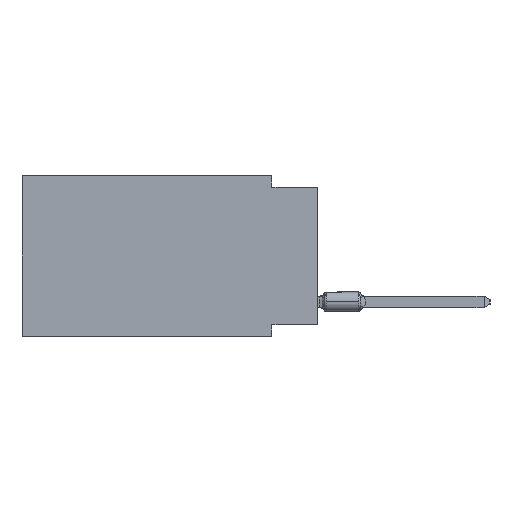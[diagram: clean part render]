
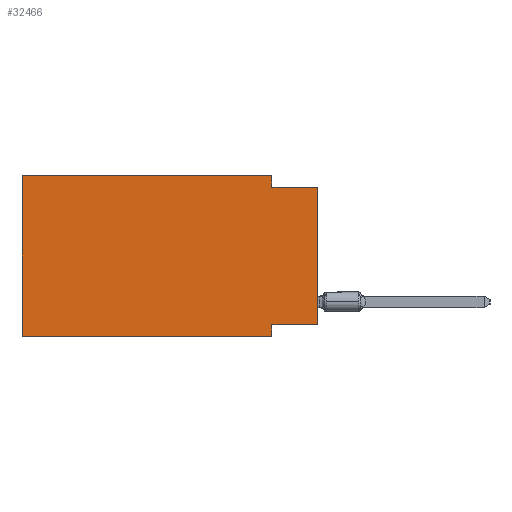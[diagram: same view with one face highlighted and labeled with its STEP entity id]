
A CAD part, left-side view. The second image highlights one B-rep face of the part: STEP entity #32466.
In plain terms, the highlighted planar face has unit normal (-1, 0, 0).
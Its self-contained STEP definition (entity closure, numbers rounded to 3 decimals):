
#559 = AXIS2_PLACEMENT_3D ( 'NONE', #15030, #29965, #12486 ) ;
#1690 = EDGE_CURVE ( 'NONE', #4900, #24685, #18037, .T. ) ;
#1785 = DIRECTION ( 'NONE',  ( 0., 0., -1. ) ) ;
#2520 = VECTOR ( 'NONE', #30578, 1000. ) ;
#2607 = LINE ( 'NONE', #26050, #9326 ) ;
#3998 = VERTEX_POINT ( 'NONE', #26127 ) ;
#4900 = VERTEX_POINT ( 'NONE', #22953 ) ;
#5017 = CARTESIAN_POINT ( 'NONE',  ( 0., 2.54, 0. ) ) ;
#5336 = ORIENTED_EDGE ( 'NONE', *, *, #18949, .F. ) ;
#5697 = ORIENTED_EDGE ( 'NONE', *, *, #27160, .T. ) ;
#6663 = DIRECTION ( 'NONE',  ( 0., -1., 0. ) ) ;
#6720 = CARTESIAN_POINT ( 'NONE',  ( 0., 2.54, -8.89 ) ) ;
#8125 = DIRECTION ( 'NONE',  ( 0., 0., 1. ) ) ;
#8494 = CARTESIAN_POINT ( 'NONE',  ( 0., 16.383, -8.89 ) ) ;
#9092 = CARTESIAN_POINT ( 'NONE',  ( 0., 2.54, -0.635 ) ) ;
#9241 = VECTOR ( 'NONE', #1785, 1000. ) ;
#9326 = VECTOR ( 'NONE', #22831, 1000. ) ;
#11205 = CARTESIAN_POINT ( 'NONE',  ( 0., 0., 0. ) ) ;
#11702 = VECTOR ( 'NONE', #21487, 1000. ) ;
#11931 = CARTESIAN_POINT ( 'NONE',  ( 0., 16.383, 0. ) ) ;
#12041 = ORIENTED_EDGE ( 'NONE', *, *, #31662, .F. ) ;
#12143 = PLANE ( 'NONE',  #559 ) ;
#12486 = DIRECTION ( 'NONE',  ( 0., 0., -1. ) ) ;
#14086 = CARTESIAN_POINT ( 'NONE',  ( 0., 0., -8.255 ) ) ;
#15030 = CARTESIAN_POINT ( 'NONE',  ( 0., 16.383, 0. ) ) ;
#15844 = VECTOR ( 'NONE', #6663, 1000. ) ;
#16137 = LINE ( 'NONE', #11205, #31351 ) ;
#16819 = CARTESIAN_POINT ( 'NONE',  ( 0., 2.54, -8.89 ) ) ;
#18037 = LINE ( 'NONE', #6720, #9241 ) ;
#18649 = CARTESIAN_POINT ( 'NONE',  ( 0., 16.383, 0. ) ) ;
#18949 = EDGE_CURVE ( 'NONE', #28218, #4900, #26963, .T. ) ;
#19326 = DIRECTION ( 'NONE',  ( 0., 1., 0. ) ) ;
#19624 = FACE_OUTER_BOUND ( 'NONE', #31236, .T. ) ;
#20350 = CARTESIAN_POINT ( 'NONE',  ( 0., 0., -8.255 ) ) ;
#21392 = DIRECTION ( 'NONE',  ( 0., 0., 1. ) ) ;
#21487 = DIRECTION ( 'NONE',  ( 0., -1., 0. ) ) ;
#21732 = VECTOR ( 'NONE', #19326, 1000. ) ;
#21872 = LINE ( 'NONE', #18649, #27008 ) ;
#22106 = LINE ( 'NONE', #11931, #2520 ) ;
#22497 = VERTEX_POINT ( 'NONE', #5017 ) ;
#22831 = DIRECTION ( 'NONE',  ( 0., 0., -1. ) ) ;
#22953 = CARTESIAN_POINT ( 'NONE',  ( 0., 2.54, -8.255 ) ) ;
#24598 = EDGE_CURVE ( 'NONE', #28218, #3998, #16137, .T. ) ;
#24685 = VERTEX_POINT ( 'NONE', #16819 ) ;
#24711 = CARTESIAN_POINT ( 'NONE',  ( 0., 16.383, -8.89 ) ) ;
#26050 = CARTESIAN_POINT ( 'NONE',  ( 0., 2.54, 0. ) ) ;
#26127 = CARTESIAN_POINT ( 'NONE',  ( 0., 0., -0.635 ) ) ;
#26963 = LINE ( 'NONE', #14086, #21732 ) ;
#27008 = VECTOR ( 'NONE', #8125, 1000. ) ;
#27160 = EDGE_CURVE ( 'NONE', #28047, #24685, #29291, .T. ) ;
#27540 = CARTESIAN_POINT ( 'NONE',  ( 0., 0., -0.635 ) ) ;
#27758 = EDGE_CURVE ( 'NONE', #29347, #22497, #22106, .T. ) ;
#28047 = VERTEX_POINT ( 'NONE', #8494 ) ;
#28129 = ORIENTED_EDGE ( 'NONE', *, *, #24598, .T. ) ;
#28218 = VERTEX_POINT ( 'NONE', #20350 ) ;
#28386 = EDGE_CURVE ( 'NONE', #28047, #29347, #21872, .T. ) ;
#29178 = ORIENTED_EDGE ( 'NONE', *, *, #31325, .F. ) ;
#29252 = ORIENTED_EDGE ( 'NONE', *, *, #28386, .F. ) ;
#29291 = LINE ( 'NONE', #24711, #11702 ) ;
#29347 = VERTEX_POINT ( 'NONE', #30048 ) ;
#29919 = LINE ( 'NONE', #27540, #15844 ) ;
#29965 = DIRECTION ( 'NONE',  ( 1., 0., 0. ) ) ;
#30048 = CARTESIAN_POINT ( 'NONE',  ( 0., 16.383, 0. ) ) ;
#30183 = VERTEX_POINT ( 'NONE', #9092 ) ;
#30578 = DIRECTION ( 'NONE',  ( 0., -1., 0. ) ) ;
#31236 = EDGE_LOOP ( 'NONE', ( #28129, #12041, #29178, #32493, #29252, #5697, #32876, #5336 ) ) ;
#31325 = EDGE_CURVE ( 'NONE', #22497, #30183, #2607, .T. ) ;
#31351 = VECTOR ( 'NONE', #21392, 1000. ) ;
#31662 = EDGE_CURVE ( 'NONE', #30183, #3998, #29919, .T. ) ;
#32466 = ADVANCED_FACE ( 'NONE', ( #19624 ), #12143, .F. ) ;
#32493 = ORIENTED_EDGE ( 'NONE', *, *, #27758, .F. ) ;
#32876 = ORIENTED_EDGE ( 'NONE', *, *, #1690, .F. ) ;
